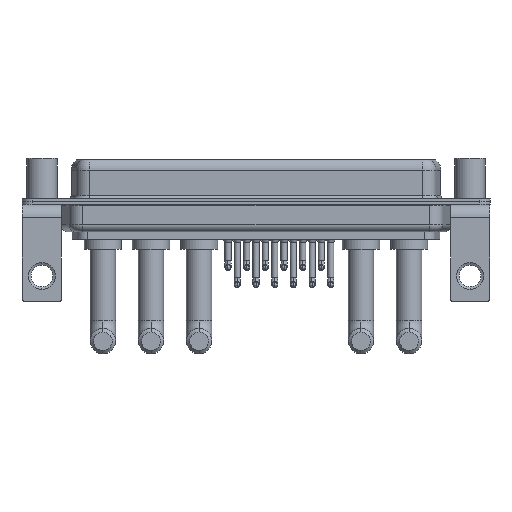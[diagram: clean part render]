
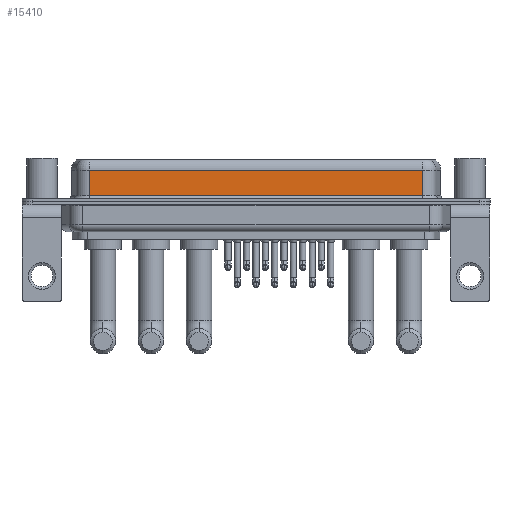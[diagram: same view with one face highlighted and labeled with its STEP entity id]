
A CAD part, front view. The second image highlights one B-rep face of the part: STEP entity #15410.
In plain terms, the highlighted planar face has unit normal (0, -1, 0).
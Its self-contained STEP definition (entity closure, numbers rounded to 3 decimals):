
#28 = EDGE_CURVE ( 'NONE', #18586, #8856, #6851, .T. ) ;
#428 = VECTOR ( 'NONE', #13847, 1000. ) ;
#478 = DIRECTION ( 'NONE',  ( 0., 1., 0. ) ) ;
#785 = CARTESIAN_POINT ( 'NONE',  ( 7.038, -3.95, 0.9 ) ) ;
#1938 = ORIENTED_EDGE ( 'NONE', *, *, #15406, .T. ) ;
#2216 = PLANE ( 'NONE',  #4743 ) ;
#2569 = FACE_OUTER_BOUND ( 'NONE', #7960, .T. ) ;
#4221 = ORIENTED_EDGE ( 'NONE', *, *, #13799, .F. ) ;
#4275 = LINE ( 'NONE', #11289, #9179 ) ;
#4743 = AXIS2_PLACEMENT_3D ( 'NONE', #9581, #478, #21532 ) ;
#6095 = EDGE_CURVE ( 'NONE', #6220, #11082, #19056, .T. ) ;
#6220 = VERTEX_POINT ( 'NONE', #16029 ) ;
#6851 = LINE ( 'NONE', #22379, #428 ) ;
#7960 = EDGE_LOOP ( 'NONE', ( #4221, #21030, #1938, #13735 ) ) ;
#8856 = VERTEX_POINT ( 'NONE', #10676 ) ;
#9179 = VECTOR ( 'NONE', #18320, 1000. ) ;
#9581 = CARTESIAN_POINT ( 'NONE',  ( 56.462, -3.95, 6.4 ) ) ;
#10676 = CARTESIAN_POINT ( 'NONE',  ( 56.462, -3.95, 0.9 ) ) ;
#11082 = VERTEX_POINT ( 'NONE', #11961 ) ;
#11289 = CARTESIAN_POINT ( 'NONE',  ( 7.038, -3.95, 6.4 ) ) ;
#11961 = CARTESIAN_POINT ( 'NONE',  ( 7.038, -3.95, 4.65 ) ) ;
#13735 = ORIENTED_EDGE ( 'NONE', *, *, #28, .T. ) ;
#13746 = DIRECTION ( 'NONE',  ( -1., 0., 0. ) ) ;
#13799 = EDGE_CURVE ( 'NONE', #6220, #8856, #13862, .T. ) ;
#13847 = DIRECTION ( 'NONE',  ( 1., 0., 0. ) ) ;
#13862 = LINE ( 'NONE', #21230, #20856 ) ;
#13961 = CARTESIAN_POINT ( 'NONE',  ( 56.462, -3.95, 4.65 ) ) ;
#15406 = EDGE_CURVE ( 'NONE', #11082, #18586, #4275, .T. ) ;
#15410 = ADVANCED_FACE ( 'NONE', ( #2569 ), #2216, .F. ) ;
#16029 = CARTESIAN_POINT ( 'NONE',  ( 56.462, -3.95, 4.65 ) ) ;
#17598 = VECTOR ( 'NONE', #13746, 1000. ) ;
#18320 = DIRECTION ( 'NONE',  ( 0., 0., -1. ) ) ;
#18586 = VERTEX_POINT ( 'NONE', #785 ) ;
#19056 = LINE ( 'NONE', #13961, #17598 ) ;
#19525 = DIRECTION ( 'NONE',  ( 0., 0., -1. ) ) ;
#20856 = VECTOR ( 'NONE', #19525, 1000. ) ;
#21030 = ORIENTED_EDGE ( 'NONE', *, *, #6095, .T. ) ;
#21230 = CARTESIAN_POINT ( 'NONE',  ( 56.462, -3.95, 6.4 ) ) ;
#21532 = DIRECTION ( 'NONE',  ( 0., 0., 1. ) ) ;
#22379 = CARTESIAN_POINT ( 'NONE',  ( 56.462, -3.95, 0.9 ) ) ;
